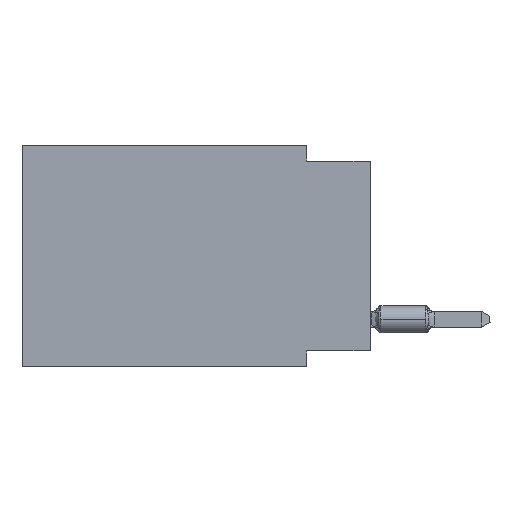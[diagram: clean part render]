
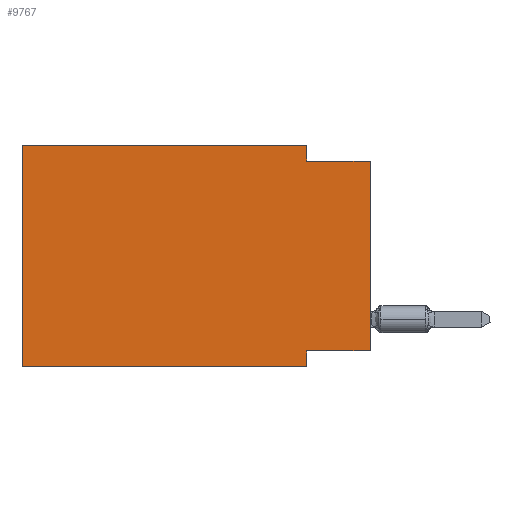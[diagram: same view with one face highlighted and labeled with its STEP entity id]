
A CAD part, left-side view. The second image highlights one B-rep face of the part: STEP entity #9767.
In plain terms, the highlighted planar face has unit normal (-1, 0, 0).
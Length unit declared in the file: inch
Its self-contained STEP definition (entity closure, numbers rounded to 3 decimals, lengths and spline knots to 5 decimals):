
#24 = VERTEX_POINT ( 'NONE', #16111 ) ;
#147 = VERTEX_POINT ( 'NONE', #16747 ) ;
#517 = EDGE_CURVE ( 'NONE', #12874, #17212, #21416, .T. ) ;
#544 = VECTOR ( 'NONE', #16097, 39.37008 ) ;
#620 = VERTEX_POINT ( 'NONE', #6273 ) ;
#964 = CARTESIAN_POINT ( 'NONE',  ( 0., 0.1, -0.325 ) ) ;
#1132 = ORIENTED_EDGE ( 'NONE', *, *, #14388, .T. ) ;
#1560 = CARTESIAN_POINT ( 'NONE',  ( 0., 0.55, -0.35 ) ) ;
#1582 = DIRECTION ( 'NONE',  ( 0., -1., 0. ) ) ;
#2301 = DIRECTION ( 'NONE',  ( 1., 0., 0. ) ) ;
#2444 = LINE ( 'NONE', #2799, #8363 ) ;
#2799 = CARTESIAN_POINT ( 'NONE',  ( 0., 0., 0. ) ) ;
#2864 = DIRECTION ( 'NONE',  ( 0., 0., 1. ) ) ;
#3816 = EDGE_CURVE ( 'NONE', #147, #12874, #17208, .T. ) ;
#3943 = EDGE_CURVE ( 'NONE', #24, #18575, #2444, .T. ) ;
#4311 = CARTESIAN_POINT ( 'NONE',  ( 0., 0.1, -0.35 ) ) ;
#4898 = CARTESIAN_POINT ( 'NONE',  ( 0., 0., -0.325 ) ) ;
#6273 = CARTESIAN_POINT ( 'NONE',  ( 0., 0.1, -0.025 ) ) ;
#6772 = ORIENTED_EDGE ( 'NONE', *, *, #15922, .F. ) ;
#8264 = VERTEX_POINT ( 'NONE', #4311 ) ;
#8315 = ORIENTED_EDGE ( 'NONE', *, *, #11974, .F. ) ;
#8363 = VECTOR ( 'NONE', #2864, 39.37008 ) ;
#8538 = AXIS2_PLACEMENT_3D ( 'NONE', #10615, #2301, #15783 ) ;
#8696 = DIRECTION ( 'NONE',  ( 0., 0., -1. ) ) ;
#9476 = EDGE_LOOP ( 'NONE', ( #13084, #8315, #21334, #21382, #11334, #1132, #6772, #12623 ) ) ;
#9767 = ADVANCED_FACE ( 'NONE', ( #18994 ), #10753, .F. ) ;
#10367 = CARTESIAN_POINT ( 'NONE',  ( 0., 0.1, 0. ) ) ;
#10615 = CARTESIAN_POINT ( 'NONE',  ( 0., 0.55, 0. ) ) ;
#10753 = PLANE ( 'NONE',  #8538 ) ;
#10772 = VECTOR ( 'NONE', #19801, 39.37008 ) ;
#10841 = CARTESIAN_POINT ( 'NONE',  ( 0., 0.55, 0. ) ) ;
#11102 = LINE ( 'NONE', #4898, #15004 ) ;
#11334 = ORIENTED_EDGE ( 'NONE', *, *, #3816, .F. ) ;
#11818 = LINE ( 'NONE', #1560, #10772 ) ;
#11974 = EDGE_CURVE ( 'NONE', #620, #18575, #17692, .T. ) ;
#12247 = CARTESIAN_POINT ( 'NONE',  ( 0., 0.55, 0. ) ) ;
#12560 = LINE ( 'NONE', #16859, #15429 ) ;
#12623 = ORIENTED_EDGE ( 'NONE', *, *, #17016, .F. ) ;
#12772 = VECTOR ( 'NONE', #15853, 39.37008 ) ;
#12874 = VERTEX_POINT ( 'NONE', #12247 ) ;
#13026 = CARTESIAN_POINT ( 'NONE',  ( 0., 0.55, 0. ) ) ;
#13084 = ORIENTED_EDGE ( 'NONE', *, *, #3943, .T. ) ;
#13140 = VECTOR ( 'NONE', #1582, 39.37008 ) ;
#14388 = EDGE_CURVE ( 'NONE', #147, #8264, #11818, .T. ) ;
#15004 = VECTOR ( 'NONE', #16985, 39.37008 ) ;
#15429 = VECTOR ( 'NONE', #8696, 39.37008 ) ;
#15536 = VECTOR ( 'NONE', #16188, 39.37008 ) ;
#15783 = DIRECTION ( 'NONE',  ( 0., 0., -1. ) ) ;
#15853 = DIRECTION ( 'NONE',  ( 0., 0., 1. ) ) ;
#15922 = EDGE_CURVE ( 'NONE', #17663, #8264, #12560, .T. ) ;
#16097 = DIRECTION ( 'NONE',  ( 0., -1., 0. ) ) ;
#16111 = CARTESIAN_POINT ( 'NONE',  ( 0., 0., -0.325 ) ) ;
#16188 = DIRECTION ( 'NONE',  ( 0., 0., -1. ) ) ;
#16747 = CARTESIAN_POINT ( 'NONE',  ( 0., 0.55, -0.35 ) ) ;
#16859 = CARTESIAN_POINT ( 'NONE',  ( 0., 0.1, -0.35 ) ) ;
#16985 = DIRECTION ( 'NONE',  ( 0., 1., 0. ) ) ;
#17016 = EDGE_CURVE ( 'NONE', #24, #17663, #11102, .T. ) ;
#17208 = LINE ( 'NONE', #10841, #12772 ) ;
#17212 = VERTEX_POINT ( 'NONE', #10367 ) ;
#17663 = VERTEX_POINT ( 'NONE', #964 ) ;
#17692 = LINE ( 'NONE', #21074, #544 ) ;
#17870 = EDGE_CURVE ( 'NONE', #17212, #620, #19650, .T. ) ;
#18575 = VERTEX_POINT ( 'NONE', #21502 ) ;
#18994 = FACE_OUTER_BOUND ( 'NONE', #9476, .T. ) ;
#19650 = LINE ( 'NONE', #21097, #15536 ) ;
#19801 = DIRECTION ( 'NONE',  ( 0., -1., 0. ) ) ;
#21074 = CARTESIAN_POINT ( 'NONE',  ( 0., 0., -0.025 ) ) ;
#21097 = CARTESIAN_POINT ( 'NONE',  ( 0., 0.1, 0. ) ) ;
#21334 = ORIENTED_EDGE ( 'NONE', *, *, #17870, .F. ) ;
#21382 = ORIENTED_EDGE ( 'NONE', *, *, #517, .F. ) ;
#21416 = LINE ( 'NONE', #13026, #13140 ) ;
#21502 = CARTESIAN_POINT ( 'NONE',  ( 0., 0., -0.025 ) ) ;
